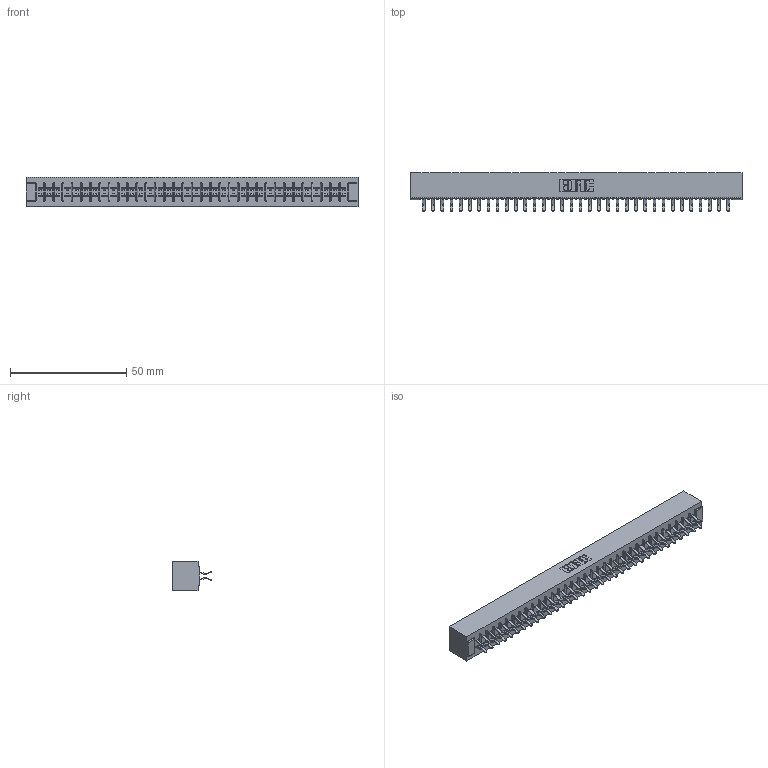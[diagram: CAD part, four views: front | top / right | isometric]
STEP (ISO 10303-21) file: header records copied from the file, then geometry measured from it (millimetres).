
FILE_DESCRIPTION (( 'STEP AP203' ), '1' );
FILE_NAME ('355-068-556-201.STEP', '2019-09-12T17:08:44', ( '' ), ( '' ), 'SwSTEP 2.0', 'SolidWorks 2016', '' );
FILE_SCHEMA (( 'CONFIG_CONTROL_DESIGN' ));
Length unit declared in the file: inch
Products named in the file (3): 305-290-001_556; 355-068-556-201; 305 Part_No Mounting
Assembly tree (69 placements, depth 2):
  355-068-556-201
    305 Part_No Mounting
    305-290-001_556  x68
Bounding box: 142.6 x 16.64 x 12.7 mm (x, y, z)
Volume: 15297.6 mm3; surface area: 19716.9 mm2
Topology: 69 solids, 69 shells, 3916 faces, 11274 edges, 7332 vertices
Faces by surface type: plane 2172, cylinder 1608, sphere 136
Entity records: 37731 total; most frequent: CARTESIAN_POINT 6244, ORIENTED_EDGE 6196, DIRECTION 6048, EDGE_CURVE 3098, VECTOR 2496, LINE 2496, VERTEX_POINT 1972, AXIS2_PLACEMENT_3D 1776
